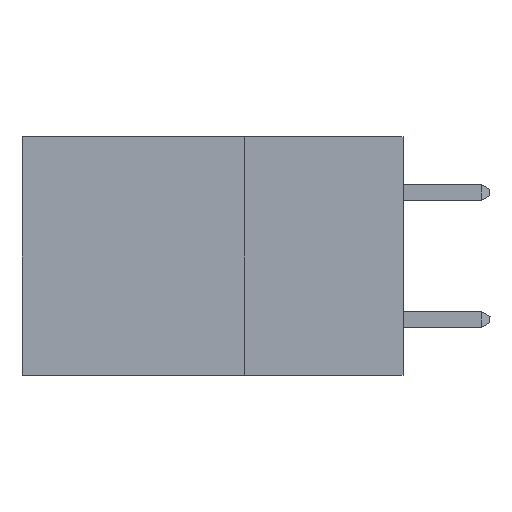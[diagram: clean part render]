
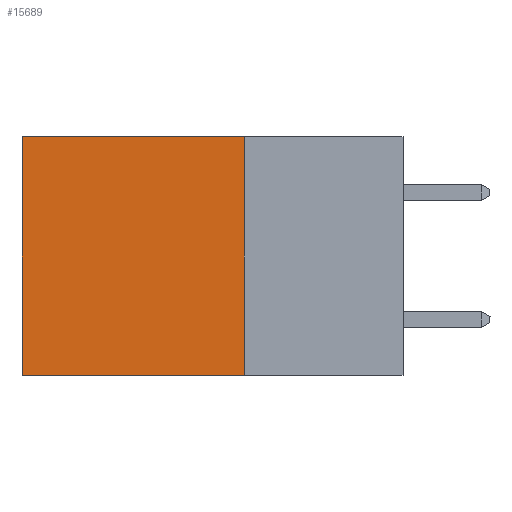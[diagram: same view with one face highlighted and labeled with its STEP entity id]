
A CAD part, left-side view. The second image highlights one B-rep face of the part: STEP entity #15689.
In plain terms, the highlighted planar face has unit normal (-1, 0, 0).
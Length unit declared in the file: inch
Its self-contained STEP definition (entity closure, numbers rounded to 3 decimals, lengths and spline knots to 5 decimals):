
#90 = VERTEX_POINT ( 'NONE', #12735 ) ;
#195 = EDGE_CURVE ( 'NONE', #9706, #90, #13815, .T. ) ;
#927 = CARTESIAN_POINT ( 'NONE',  ( 0.2875, 0.25, -0.375 ) ) ;
#1529 = VECTOR ( 'NONE', #7490, 39.37008 ) ;
#1740 = CARTESIAN_POINT ( 'NONE',  ( 0.2875, 0.25, 0. ) ) ;
#1929 = LINE ( 'NONE', #6047, #1529 ) ;
#2070 = DIRECTION ( 'NONE',  ( 0., 0., -1. ) ) ;
#3023 = ORIENTED_EDGE ( 'NONE', *, *, #9296, .T. ) ;
#4655 = VECTOR ( 'NONE', #6429, 39.37008 ) ;
#4976 = CARTESIAN_POINT ( 'NONE',  ( 0.2875, 0.6, 0. ) ) ;
#5131 = DIRECTION ( 'NONE',  ( 0., 0., -1. ) ) ;
#5855 = EDGE_CURVE ( 'NONE', #7661, #11612, #1929, .T. ) ;
#5897 = DIRECTION ( 'NONE',  ( 1., 0., 0. ) ) ;
#6047 = CARTESIAN_POINT ( 'NONE',  ( 0.2875, 0.25, 0. ) ) ;
#6429 = DIRECTION ( 'NONE',  ( 0., 1., 0. ) ) ;
#7447 = PLANE ( 'NONE',  #11974 ) ;
#7490 = DIRECTION ( 'NONE',  ( 0., 1., 0. ) ) ;
#7661 = VERTEX_POINT ( 'NONE', #1740 ) ;
#7703 = CARTESIAN_POINT ( 'NONE',  ( 0.2875, 0.25, -0.375 ) ) ;
#7872 = EDGE_LOOP ( 'NONE', ( #3023, #14322, #16088, #10463 ) ) ;
#7986 = EDGE_CURVE ( 'NONE', #7661, #9706, #16438, .T. ) ;
#8799 = FACE_OUTER_BOUND ( 'NONE', #7872, .T. ) ;
#8963 = CARTESIAN_POINT ( 'NONE',  ( 0.2875, 0.25, -0.375 ) ) ;
#9277 = LINE ( 'NONE', #16767, #10315 ) ;
#9296 = EDGE_CURVE ( 'NONE', #11612, #90, #9277, .T. ) ;
#9706 = VERTEX_POINT ( 'NONE', #12378 ) ;
#10050 = DIRECTION ( 'NONE',  ( 0., 0., -1. ) ) ;
#10315 = VECTOR ( 'NONE', #10050, 39.37008 ) ;
#10463 = ORIENTED_EDGE ( 'NONE', *, *, #5855, .T. ) ;
#11612 = VERTEX_POINT ( 'NONE', #4976 ) ;
#11974 = AXIS2_PLACEMENT_3D ( 'NONE', #927, #5897, #2070 ) ;
#12378 = CARTESIAN_POINT ( 'NONE',  ( 0.2875, 0.25, -0.375 ) ) ;
#12735 = CARTESIAN_POINT ( 'NONE',  ( 0.2875, 0.6, -0.375 ) ) ;
#13815 = LINE ( 'NONE', #7703, #4655 ) ;
#14322 = ORIENTED_EDGE ( 'NONE', *, *, #195, .F. ) ;
#15689 = ADVANCED_FACE ( 'NONE', ( #8799 ), #7447, .F. ) ;
#15847 = VECTOR ( 'NONE', #5131, 39.37008 ) ;
#16088 = ORIENTED_EDGE ( 'NONE', *, *, #7986, .F. ) ;
#16438 = LINE ( 'NONE', #8963, #15847 ) ;
#16767 = CARTESIAN_POINT ( 'NONE',  ( 0.2875, 0.6, -0.375 ) ) ;
